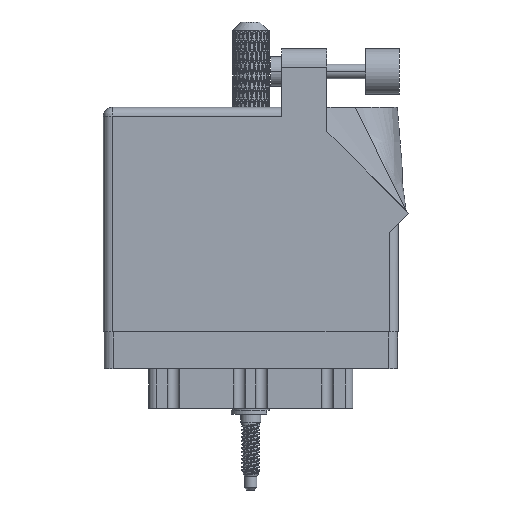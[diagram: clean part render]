
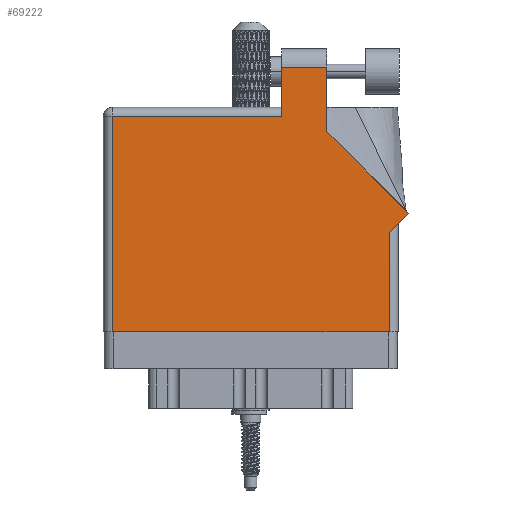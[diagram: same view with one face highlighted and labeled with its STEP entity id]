
A CAD part, front view. The second image highlights one B-rep face of the part: STEP entity #69222.
In plain terms, the highlighted face is planar.
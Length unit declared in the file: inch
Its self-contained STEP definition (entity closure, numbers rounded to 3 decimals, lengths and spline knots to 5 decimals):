
#283 = DIRECTION ( 'NONE',  ( -1., 0., 0. ) ) ;
#1000 = LINE ( 'NONE', #25356, #52860 ) ;
#2892 = DIRECTION ( 'NONE',  ( -1., 0., 0. ) ) ;
#4597 = VECTOR ( 'NONE', #41463, 39.37008 ) ;
#11335 = CARTESIAN_POINT ( 'NONE',  ( 1.948, 0.675, 0. ) ) ;
#14618 = CARTESIAN_POINT ( 'NONE',  ( 0., 1.53, 0. ) ) ;
#15725 = CARTESIAN_POINT ( 'NONE',  ( 1.524, 1.36442, 0. ) ) ;
#15945 = VECTOR ( 'NONE', #2892, 39.37008 ) ;
#16271 = LINE ( 'NONE', #88611, #103209 ) ;
#19869 = VERTEX_POINT ( 'NONE', #66727 ) ;
#21773 = VECTOR ( 'NONE', #70385, 39.37008 ) ;
#21806 = ORIENTED_EDGE ( 'NONE', *, *, #27461, .T. ) ;
#23335 = ORIENTED_EDGE ( 'NONE', *, *, #56529, .T. ) ;
#23794 = LINE ( 'NONE', #71863, #97725 ) ;
#24002 = EDGE_CURVE ( 'NONE', #100384, #19869, #16271, .T. ) ;
#25356 = CARTESIAN_POINT ( 'NONE',  ( 0., 1.468, 0. ) ) ;
#26111 = ORIENTED_EDGE ( 'NONE', *, *, #33771, .T. ) ;
#27461 = EDGE_CURVE ( 'NONE', #95077, #62466, #59930, .T. ) ;
#27725 = LINE ( 'NONE', #75282, #90673 ) ;
#29625 = CARTESIAN_POINT ( 'NONE',  ( 1.217, 1.805, 0. ) ) ;
#31657 = EDGE_CURVE ( 'NONE', #62466, #97634, #27725, .T. ) ;
#33771 = EDGE_CURVE ( 'NONE', #45464, #95077, #39493, .T. ) ;
#34311 = EDGE_CURVE ( 'NONE', #97634, #52540, #1000, .T. ) ;
#36504 = CARTESIAN_POINT ( 'NONE',  ( 0.062, 0., 0. ) ) ;
#36695 = DIRECTION ( 'NONE',  ( 0., -1., 0. ) ) ;
#37617 = AXIS2_PLACEMENT_3D ( 'NONE', #14618, #90603, #283 ) ;
#37635 = CARTESIAN_POINT ( 'NONE',  ( 1.217, 1.468, 0. ) ) ;
#39493 = LINE ( 'NONE', #15725, #46314 ) ;
#41463 = DIRECTION ( 'NONE',  ( 0., -1., 0. ) ) ;
#44108 = CARTESIAN_POINT ( 'NONE',  ( 1.217, 1.805, 0. ) ) ;
#44473 = EDGE_CURVE ( 'NONE', #52540, #100384, #99531, .T. ) ;
#45464 = VERTEX_POINT ( 'NONE', #59770 ) ;
#45526 = VERTEX_POINT ( 'NONE', #59245 ) ;
#46314 = VECTOR ( 'NONE', #73800, 39.37008 ) ;
#51083 = EDGE_LOOP ( 'NONE', ( #26111, #21806, #62723, #66646, #51562, #66351, #100127, #23335, #76257 ) ) ;
#51562 = ORIENTED_EDGE ( 'NONE', *, *, #44473, .T. ) ;
#52540 = VERTEX_POINT ( 'NONE', #96999 ) ;
#52860 = VECTOR ( 'NONE', #97183, 39.37008 ) ;
#54114 = DIRECTION ( 'NONE',  ( 0., 1., 0. ) ) ;
#54502 = LINE ( 'NONE', #61908, #21773 ) ;
#55448 = DIRECTION ( 'NONE',  ( 0.707, 0.707, 0. ) ) ;
#56529 = EDGE_CURVE ( 'NONE', #75624, #45526, #23794, .T. ) ;
#56607 = CARTESIAN_POINT ( 'NONE',  ( 1.948, 0.737, 0. ) ) ;
#58839 = EDGE_CURVE ( 'NONE', #45526, #45464, #54502, .T. ) ;
#59245 = CARTESIAN_POINT ( 'NONE',  ( 2.08071, 0.80771, 0. ) ) ;
#59357 = CARTESIAN_POINT ( 'NONE',  ( 0.062, 0., 0. ) ) ;
#59770 = CARTESIAN_POINT ( 'NONE',  ( 1.524, 1.36442, 0. ) ) ;
#59930 = LINE ( 'NONE', #44108, #15945 ) ;
#61908 = CARTESIAN_POINT ( 'NONE',  ( 2.08071, 0.80771, 0. ) ) ;
#62466 = VERTEX_POINT ( 'NONE', #29625 ) ;
#62723 = ORIENTED_EDGE ( 'NONE', *, *, #31657, .T. ) ;
#66351 = ORIENTED_EDGE ( 'NONE', *, *, #24002, .T. ) ;
#66646 = ORIENTED_EDGE ( 'NONE', *, *, #34311, .T. ) ;
#66727 = CARTESIAN_POINT ( 'NONE',  ( 1.948, 0., 0. ) ) ;
#67042 = CARTESIAN_POINT ( 'NONE',  ( 1.524, 1.805, 0. ) ) ;
#69222 = ADVANCED_FACE ( 'NONE', ( #102853 ), #94911, .F. ) ;
#70385 = DIRECTION ( 'NONE',  ( -0.707, 0.707, 0. ) ) ;
#71863 = CARTESIAN_POINT ( 'NONE',  ( 2.01, 0.737, 0. ) ) ;
#72484 = LINE ( 'NONE', #56607, #79675 ) ;
#72783 = DIRECTION ( 'NONE',  ( 1., 0., 0. ) ) ;
#73800 = DIRECTION ( 'NONE',  ( 0., 1., 0. ) ) ;
#75282 = CARTESIAN_POINT ( 'NONE',  ( 1.217, 1.53, 0. ) ) ;
#75624 = VERTEX_POINT ( 'NONE', #11335 ) ;
#76257 = ORIENTED_EDGE ( 'NONE', *, *, #58839, .T. ) ;
#79675 = VECTOR ( 'NONE', #54114, 39.37008 ) ;
#88611 = CARTESIAN_POINT ( 'NONE',  ( 0., 0., 0. ) ) ;
#90603 = DIRECTION ( 'NONE',  ( 0., 0., -1. ) ) ;
#90673 = VECTOR ( 'NONE', #36695, 39.37008 ) ;
#94911 = PLANE ( 'NONE',  #37617 ) ;
#95077 = VERTEX_POINT ( 'NONE', #67042 ) ;
#96999 = CARTESIAN_POINT ( 'NONE',  ( 0.062, 1.468, 0. ) ) ;
#97183 = DIRECTION ( 'NONE',  ( -1., 0., 0. ) ) ;
#97634 = VERTEX_POINT ( 'NONE', #37635 ) ;
#97725 = VECTOR ( 'NONE', #55448, 39.37008 ) ;
#99531 = LINE ( 'NONE', #59357, #4597 ) ;
#100127 = ORIENTED_EDGE ( 'NONE', *, *, #103675, .T. ) ;
#100384 = VERTEX_POINT ( 'NONE', #36504 ) ;
#102853 = FACE_OUTER_BOUND ( 'NONE', #51083, .T. ) ;
#103209 = VECTOR ( 'NONE', #72783, 39.37008 ) ;
#103675 = EDGE_CURVE ( 'NONE', #19869, #75624, #72484, .T. ) ;
